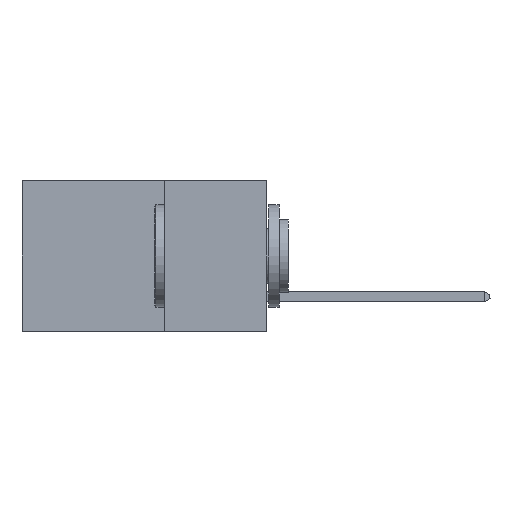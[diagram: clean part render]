
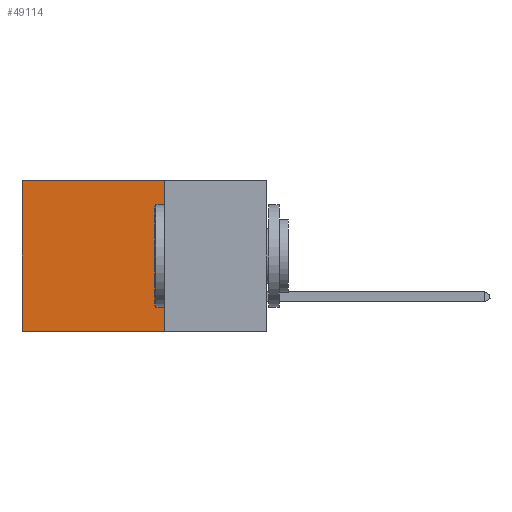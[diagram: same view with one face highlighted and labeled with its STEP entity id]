
A CAD part, left-side view. The second image highlights one B-rep face of the part: STEP entity #49114.
In plain terms, the highlighted planar face has unit normal (-1, 0, 0).
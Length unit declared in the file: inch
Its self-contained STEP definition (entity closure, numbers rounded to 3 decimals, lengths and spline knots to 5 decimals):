
#707 = CARTESIAN_POINT ( 'NONE',  ( 0.2875, 0.25, -0.37 ) ) ;
#1841 = LINE ( 'NONE', #36902, #13646 ) ;
#3316 = DIRECTION ( 'NONE',  ( 0., 1., 0. ) ) ;
#6238 = CARTESIAN_POINT ( 'NONE',  ( 0.2875, 0.6, -0.37 ) ) ;
#9910 = CARTESIAN_POINT ( 'NONE',  ( 0.2875, 0.25, 0. ) ) ;
#12355 = EDGE_CURVE ( 'NONE', #40812, #43192, #41782, .T. ) ;
#12738 = VECTOR ( 'NONE', #3316, 39.37008 ) ;
#13646 = VECTOR ( 'NONE', #18486, 39.37008 ) ;
#15043 = CARTESIAN_POINT ( 'NONE',  ( 0.2875, 0.25, 0. ) ) ;
#16964 = DIRECTION ( 'NONE',  ( 0., 0., -1. ) ) ;
#17556 = LINE ( 'NONE', #27081, #35335 ) ;
#17922 = DIRECTION ( 'NONE',  ( 0., 0., -1. ) ) ;
#18486 = DIRECTION ( 'NONE',  ( 0., 1., 0. ) ) ;
#23753 = DIRECTION ( 'NONE',  ( 0., 0., -1. ) ) ;
#24188 = ORIENTED_EDGE ( 'NONE', *, *, #25684, .T. ) ;
#24238 = DIRECTION ( 'NONE',  ( 1., 0., 0. ) ) ;
#24764 = VERTEX_POINT ( 'NONE', #6238 ) ;
#25496 = ORIENTED_EDGE ( 'NONE', *, *, #39742, .F. ) ;
#25684 = EDGE_CURVE ( 'NONE', #43192, #24764, #17556, .T. ) ;
#27081 = CARTESIAN_POINT ( 'NONE',  ( 0.2875, 0.6, 0. ) ) ;
#29496 = EDGE_LOOP ( 'NONE', ( #24188, #44318, #25496, #39280 ) ) ;
#32025 = PLANE ( 'NONE',  #40123 ) ;
#32862 = VERTEX_POINT ( 'NONE', #707 ) ;
#35335 = VECTOR ( 'NONE', #23753, 39.37008 ) ;
#35995 = CARTESIAN_POINT ( 'NONE',  ( 0.2875, 0.25, 0. ) ) ;
#36902 = CARTESIAN_POINT ( 'NONE',  ( 0.2875, 0.25, -0.37 ) ) ;
#37984 = FACE_OUTER_BOUND ( 'NONE', #29496, .T. ) ;
#39280 = ORIENTED_EDGE ( 'NONE', *, *, #12355, .T. ) ;
#39679 = CARTESIAN_POINT ( 'NONE',  ( 0.2875, 0.25, 0. ) ) ;
#39742 = EDGE_CURVE ( 'NONE', #40812, #32862, #42182, .T. ) ;
#40123 = AXIS2_PLACEMENT_3D ( 'NONE', #39679, #24238, #16964 ) ;
#40812 = VERTEX_POINT ( 'NONE', #9910 ) ;
#41782 = LINE ( 'NONE', #15043, #12738 ) ;
#42182 = LINE ( 'NONE', #35995, #42809 ) ;
#42809 = VECTOR ( 'NONE', #17922, 39.37008 ) ;
#43192 = VERTEX_POINT ( 'NONE', #43796 ) ;
#43796 = CARTESIAN_POINT ( 'NONE',  ( 0.2875, 0.6, 0. ) ) ;
#44318 = ORIENTED_EDGE ( 'NONE', *, *, #48718, .F. ) ;
#48718 = EDGE_CURVE ( 'NONE', #32862, #24764, #1841, .T. ) ;
#49114 = ADVANCED_FACE ( 'NONE', ( #37984 ), #32025, .F. ) ;
